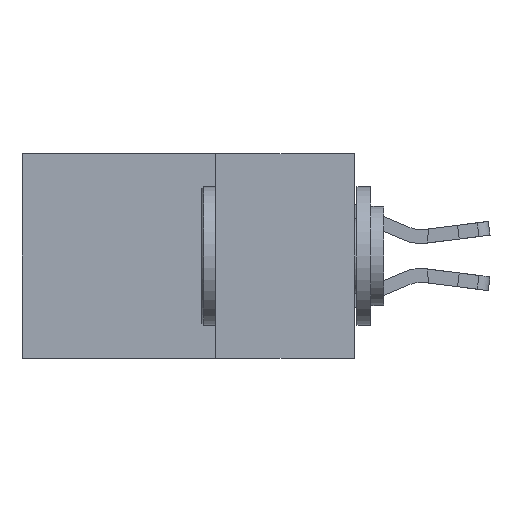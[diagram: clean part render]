
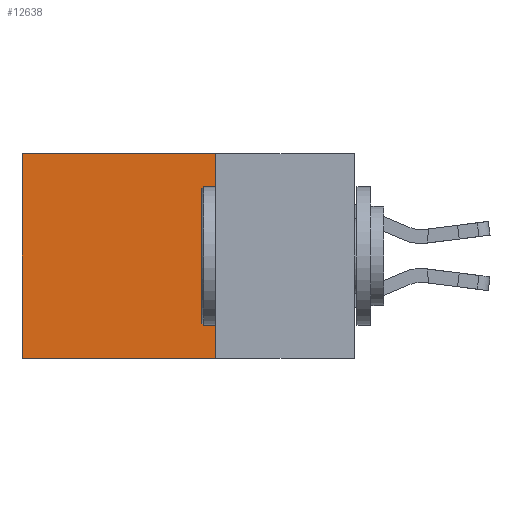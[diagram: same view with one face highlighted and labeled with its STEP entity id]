
A CAD part, left-side view. The second image highlights one B-rep face of the part: STEP entity #12638.
In plain terms, the highlighted planar face has unit normal (-1, 0, 0).
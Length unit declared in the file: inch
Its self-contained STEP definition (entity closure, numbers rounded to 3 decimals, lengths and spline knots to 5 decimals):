
#279 = DIRECTION ( 'NONE',  ( 0., 0., -1. ) ) ;
#627 = CARTESIAN_POINT ( 'NONE',  ( 0.298, 0.6, 0. ) ) ;
#793 = VECTOR ( 'NONE', #5559, 39.37008 ) ;
#1920 = CARTESIAN_POINT ( 'NONE',  ( 0.298, 0.25, -0.37 ) ) ;
#2298 = VECTOR ( 'NONE', #5319, 39.37008 ) ;
#3001 = VERTEX_POINT ( 'NONE', #12593 ) ;
#3862 = CARTESIAN_POINT ( 'NONE',  ( 0.298, 0.25, 0. ) ) ;
#4976 = EDGE_CURVE ( 'NONE', #3001, #10110, #20773, .T. ) ;
#5054 = PLANE ( 'NONE',  #8535 ) ;
#5319 = DIRECTION ( 'NONE',  ( 0., 1., 0. ) ) ;
#5559 = DIRECTION ( 'NONE',  ( 0., 0., -1. ) ) ;
#6217 = ORIENTED_EDGE ( 'NONE', *, *, #7782, .F. ) ;
#7233 = VECTOR ( 'NONE', #10201, 39.37008 ) ;
#7494 = EDGE_CURVE ( 'NONE', #10110, #16495, #12161, .T. ) ;
#7772 = ORIENTED_EDGE ( 'NONE', *, *, #7494, .T. ) ;
#7782 = EDGE_CURVE ( 'NONE', #3001, #13172, #14803, .T. ) ;
#8535 = AXIS2_PLACEMENT_3D ( 'NONE', #20559, #10361, #279 ) ;
#9156 = FACE_OUTER_BOUND ( 'NONE', #15364, .T. ) ;
#10110 = VERTEX_POINT ( 'NONE', #627 ) ;
#10201 = DIRECTION ( 'NONE',  ( 0., 1., 0. ) ) ;
#10361 = DIRECTION ( 'NONE',  ( 1., 0., 0. ) ) ;
#11300 = LINE ( 'NONE', #1920, #2298 ) ;
#11614 = CARTESIAN_POINT ( 'NONE',  ( 0.298, 0.25, -0.37 ) ) ;
#12161 = LINE ( 'NONE', #18342, #17220 ) ;
#12593 = CARTESIAN_POINT ( 'NONE',  ( 0.298, 0.25, 0. ) ) ;
#12638 = ADVANCED_FACE ( 'NONE', ( #9156 ), #5054, .F. ) ;
#13172 = VERTEX_POINT ( 'NONE', #11614 ) ;
#14768 = ORIENTED_EDGE ( 'NONE', *, *, #4976, .T. ) ;
#14803 = LINE ( 'NONE', #3862, #793 ) ;
#15364 = EDGE_LOOP ( 'NONE', ( #7772, #15974, #6217, #14768 ) ) ;
#15974 = ORIENTED_EDGE ( 'NONE', *, *, #16856, .F. ) ;
#16495 = VERTEX_POINT ( 'NONE', #21499 ) ;
#16856 = EDGE_CURVE ( 'NONE', #13172, #16495, #11300, .T. ) ;
#17220 = VECTOR ( 'NONE', #20057, 39.37008 ) ;
#18342 = CARTESIAN_POINT ( 'NONE',  ( 0.298, 0.6, 0. ) ) ;
#20057 = DIRECTION ( 'NONE',  ( 0., 0., -1. ) ) ;
#20559 = CARTESIAN_POINT ( 'NONE',  ( 0.298, 0.25, 0. ) ) ;
#20773 = LINE ( 'NONE', #20997, #7233 ) ;
#20997 = CARTESIAN_POINT ( 'NONE',  ( 0.298, 0.25, 0. ) ) ;
#21499 = CARTESIAN_POINT ( 'NONE',  ( 0.298, 0.6, -0.37 ) ) ;
